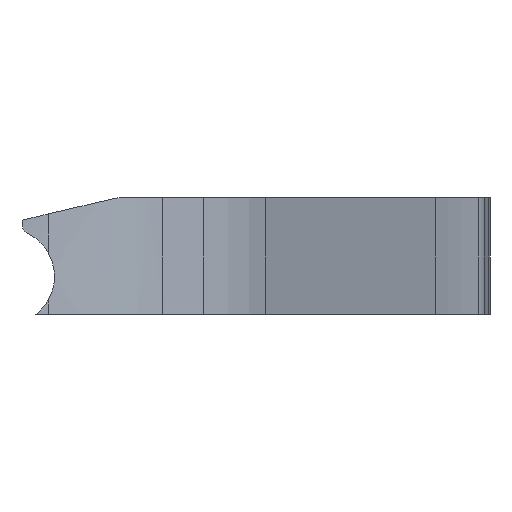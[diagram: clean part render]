
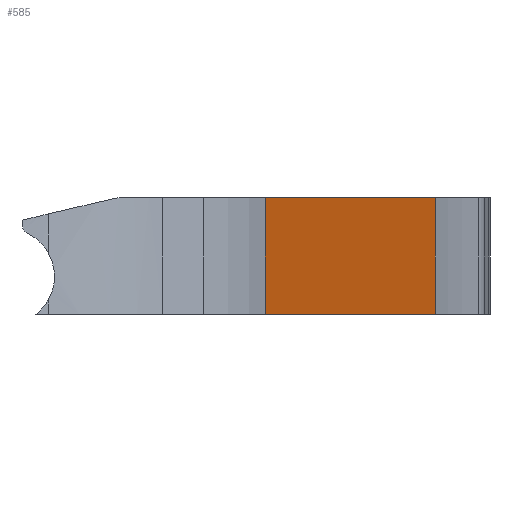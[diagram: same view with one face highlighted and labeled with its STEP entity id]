
A CAD part, left-side view. The second image highlights one B-rep face of the part: STEP entity #585.
In plain terms, the highlighted planar face has unit normal (-0.408, -0.913, 0).
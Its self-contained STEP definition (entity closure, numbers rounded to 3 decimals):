
#30=PLANE('',#637);
#48=FACE_OUTER_BOUND('',#80,.T.);
#80=EDGE_LOOP('',(#400,#401,#402,#403));
#114=LINE('',#886,#166);
#115=LINE('',#889,#167);
#116=LINE('',#891,#168);
#117=LINE('',#892,#169);
#166=VECTOR('',#712,10.);
#167=VECTOR('',#715,10.);
#168=VECTOR('',#716,10.);
#169=VECTOR('',#717,10.);
#246=VERTEX_POINT('',#882);
#247=VERTEX_POINT('',#884);
#248=VERTEX_POINT('',#888);
#249=VERTEX_POINT('',#890);
#308=EDGE_CURVE('',#247,#246,#114,.T.);
#309=EDGE_CURVE('',#248,#247,#115,.F.);
#310=EDGE_CURVE('',#249,#248,#116,.T.);
#311=EDGE_CURVE('',#246,#249,#117,.T.);
#400=ORIENTED_EDGE('',*,*,#308,.F.);
#401=ORIENTED_EDGE('',*,*,#309,.F.);
#402=ORIENTED_EDGE('',*,*,#310,.F.);
#403=ORIENTED_EDGE('',*,*,#311,.F.);
#585=ADVANCED_FACE('',(#48),#30,.F.);
#637=AXIS2_PLACEMENT_3D('',#887,#713,#714);
#712=DIRECTION('',(0.,0.,-1.));
#713=DIRECTION('center_axis',(0.408,0.913,0.));
#714=DIRECTION('ref_axis',(0.913,-0.408,0.));
#715=DIRECTION('',(-0.913,0.408,0.));
#716=DIRECTION('',(0.,0.,1.));
#717=DIRECTION('',(-0.913,0.408,0.));
#882=CARTESIAN_POINT('',(52.921,1.492,0.));
#884=CARTESIAN_POINT('',(52.921,1.492,11.85));
#886=CARTESIAN_POINT('',(52.921,1.492,12.05));
#887=CARTESIAN_POINT('Origin',(9.427,20.907,12.05));
#888=CARTESIAN_POINT('',(14.293,18.735,11.85));
#889=CARTESIAN_POINT('',(26.568,13.256,11.85));
#890=CARTESIAN_POINT('',(14.293,18.735,0.));
#891=CARTESIAN_POINT('',(14.293,18.735,12.05));
#892=CARTESIAN_POINT('',(41.799,6.457,0.));
